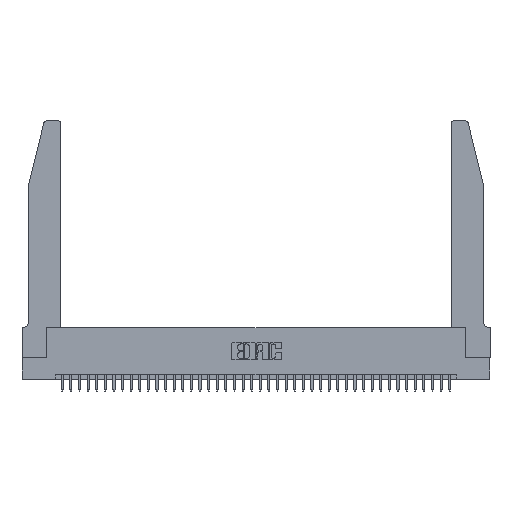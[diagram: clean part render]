
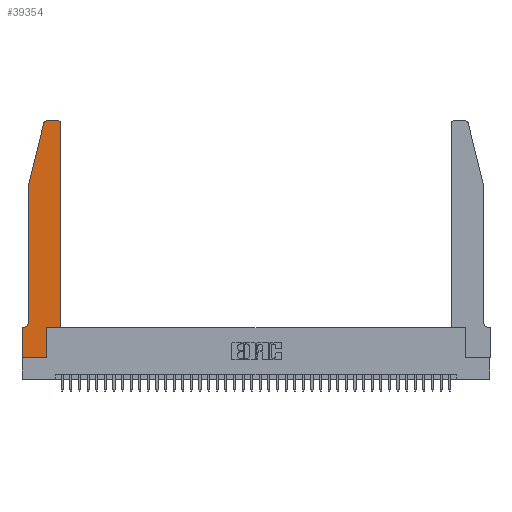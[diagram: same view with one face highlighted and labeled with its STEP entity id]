
A CAD part, top view. The second image highlights one B-rep face of the part: STEP entity #39354.
In plain terms, the highlighted planar face has unit normal (0, 0, 1).
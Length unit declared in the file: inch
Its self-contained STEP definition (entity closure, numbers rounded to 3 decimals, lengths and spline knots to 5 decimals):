
#52 = CARTESIAN_POINT ( 'NONE',  ( 0.4505, 2.72, 0.37 ) ) ;
#160 = VECTOR ( 'NONE', #38831, 39.37008 ) ;
#640 = CARTESIAN_POINT ( 'NONE',  ( 0., 0., 0.37 ) ) ;
#1344 = EDGE_CURVE ( 'NONE', #25017, #6394, #32890, .T. ) ;
#1852 = EDGE_CURVE ( 'NONE', #9838, #25017, #10891, .T. ) ;
#1958 = VERTEX_POINT ( 'NONE', #5887 ) ;
#1980 = CARTESIAN_POINT ( 'NONE',  ( 0.4505, 0.35, 0.37 ) ) ;
#2454 = EDGE_CURVE ( 'NONE', #7672, #1958, #29952, .T. ) ;
#2679 = VECTOR ( 'NONE', #15431, 39.37008 ) ;
#3601 = CIRCLE ( 'NONE', #31686, 0.07 ) ;
#4180 = CARTESIAN_POINT ( 'NONE',  ( 0.25487, 2.72718, 0.37 ) ) ;
#4517 = LINE ( 'NONE', #11717, #35699 ) ;
#4540 = VERTEX_POINT ( 'NONE', #34267 ) ;
#4733 = CARTESIAN_POINT ( 'NONE',  ( 0., 0., 0.37 ) ) ;
#5561 = ORIENTED_EDGE ( 'NONE', *, *, #21082, .T. ) ;
#5887 = CARTESIAN_POINT ( 'NONE',  ( 0.2865, 0.35, 0.37 ) ) ;
#6394 = VERTEX_POINT ( 'NONE', #34773 ) ;
#6833 = ORIENTED_EDGE ( 'NONE', *, *, #37310, .T. ) ;
#6899 = ORIENTED_EDGE ( 'NONE', *, *, #2454, .T. ) ;
#6963 = CARTESIAN_POINT ( 'NONE',  ( 0.0755, 0.35, 0.37 ) ) ;
#7026 = DIRECTION ( 'NONE',  ( 0., 0., 1. ) ) ;
#7358 = DIRECTION ( 'NONE',  ( 0., 1., 0. ) ) ;
#7595 = VECTOR ( 'NONE', #39859, 39.37008 ) ;
#7672 = VERTEX_POINT ( 'NONE', #20774 ) ;
#7779 = VERTEX_POINT ( 'NONE', #36975 ) ;
#7908 = EDGE_LOOP ( 'NONE', ( #13437, #30559, #15495, #39359, #20787, #9068, #5561, #25976, #6899, #21098, #26045, #6833 ) ) ;
#8814 = VECTOR ( 'NONE', #17128, 39.37008 ) ;
#9041 = DIRECTION ( 'NONE',  ( 1., 0., 0. ) ) ;
#9068 = ORIENTED_EDGE ( 'NONE', *, *, #19324, .T. ) ;
#9171 = CARTESIAN_POINT ( 'NONE',  ( 0.4205, 2.72, 0.37 ) ) ;
#9838 = VERTEX_POINT ( 'NONE', #30377 ) ;
#10891 = CIRCLE ( 'NONE', #25066, 0.03 ) ;
#11016 = AXIS2_PLACEMENT_3D ( 'NONE', #9171, #28280, #24979 ) ;
#11222 = DIRECTION ( 'NONE',  ( 0., 0., -1. ) ) ;
#11717 = CARTESIAN_POINT ( 'NONE',  ( 0.4505, 0.35, 0.37 ) ) ;
#11773 = VERTEX_POINT ( 'NONE', #640 ) ;
#12362 = CIRCLE ( 'NONE', #11016, 0.03 ) ;
#13437 = ORIENTED_EDGE ( 'NONE', *, *, #26043, .T. ) ;
#13748 = VECTOR ( 'NONE', #23115, 39.37008 ) ;
#13892 = VECTOR ( 'NONE', #7358, 39.37008 ) ;
#14963 = EDGE_CURVE ( 'NONE', #4540, #35658, #40292, .T. ) ;
#15431 = DIRECTION ( 'NONE',  ( -0.239, -0.971, 0. ) ) ;
#15495 = ORIENTED_EDGE ( 'NONE', *, *, #1344, .T. ) ;
#15550 = VECTOR ( 'NONE', #21327, 39.37008 ) ;
#15794 = CARTESIAN_POINT ( 'NONE',  ( 0.0755, 2., 0.37 ) ) ;
#16838 = CARTESIAN_POINT ( 'NONE',  ( 0., 0.35, 0.37 ) ) ;
#17128 = DIRECTION ( 'NONE',  ( 1., 0., 0. ) ) ;
#18031 = LINE ( 'NONE', #6963, #38524 ) ;
#18348 = VERTEX_POINT ( 'NONE', #18523 ) ;
#18523 = CARTESIAN_POINT ( 'NONE',  ( 0.0055, 0.35, 0.37 ) ) ;
#19031 = VERTEX_POINT ( 'NONE', #32284 ) ;
#19324 = EDGE_CURVE ( 'NONE', #18348, #19031, #18031, .T. ) ;
#19551 = DIRECTION ( 'NONE',  ( 1., 0., 0. ) ) ;
#20001 = CARTESIAN_POINT ( 'NONE',  ( 0.2605, 2.75, 0.37 ) ) ;
#20774 = CARTESIAN_POINT ( 'NONE',  ( 0.2865, 0., 0.37 ) ) ;
#20787 = ORIENTED_EDGE ( 'NONE', *, *, #38173, .T. ) ;
#21021 = CARTESIAN_POINT ( 'NONE',  ( 0.0055, 0.42, 0.37 ) ) ;
#21082 = EDGE_CURVE ( 'NONE', #19031, #11773, #25913, .T. ) ;
#21098 = ORIENTED_EDGE ( 'NONE', *, *, #39048, .T. ) ;
#21327 = DIRECTION ( 'NONE',  ( 0., -1., 0. ) ) ;
#22355 = CARTESIAN_POINT ( 'NONE',  ( 0.2865, 0.35, 0.37 ) ) ;
#23115 = DIRECTION ( 'NONE',  ( 0., -1., 0. ) ) ;
#23856 = LINE ( 'NONE', #33466, #15550 ) ;
#24187 = AXIS2_PLACEMENT_3D ( 'NONE', #16838, #7026, #19551 ) ;
#24648 = DIRECTION ( 'NONE',  ( 1., 0., 0. ) ) ;
#24979 = DIRECTION ( 'NONE',  ( 1., 0., 0. ) ) ;
#25017 = VERTEX_POINT ( 'NONE', #4180 ) ;
#25066 = AXIS2_PLACEMENT_3D ( 'NONE', #25802, #35178, #9041 ) ;
#25802 = CARTESIAN_POINT ( 'NONE',  ( 0.284, 2.72, 0.37 ) ) ;
#25913 = LINE ( 'NONE', #4733, #13748 ) ;
#25976 = ORIENTED_EDGE ( 'NONE', *, *, #34323, .T. ) ;
#26003 = CARTESIAN_POINT ( 'NONE',  ( 0., 0., 0.37 ) ) ;
#26043 = EDGE_CURVE ( 'NONE', #30012, #9838, #34295, .T. ) ;
#26045 = ORIENTED_EDGE ( 'NONE', *, *, #14963, .T. ) ;
#27066 = DIRECTION ( 'NONE',  ( -1., 0., 0. ) ) ;
#28280 = DIRECTION ( 'NONE',  ( 0., 0., 1. ) ) ;
#29811 = CARTESIAN_POINT ( 'NONE',  ( 0.4205, 2.75, 0.37 ) ) ;
#29952 = LINE ( 'NONE', #22355, #13892 ) ;
#30012 = VERTEX_POINT ( 'NONE', #29811 ) ;
#30047 = EDGE_CURVE ( 'NONE', #6394, #7779, #23856, .T. ) ;
#30377 = CARTESIAN_POINT ( 'NONE',  ( 0.284, 2.75, 0.37 ) ) ;
#30559 = ORIENTED_EDGE ( 'NONE', *, *, #1852, .T. ) ;
#31686 = AXIS2_PLACEMENT_3D ( 'NONE', #21021, #11222, #27066 ) ;
#32284 = CARTESIAN_POINT ( 'NONE',  ( 0., 0.35, 0.37 ) ) ;
#32890 = LINE ( 'NONE', #15794, #2679 ) ;
#33466 = CARTESIAN_POINT ( 'NONE',  ( 0.0755, 2., 0.37 ) ) ;
#34267 = CARTESIAN_POINT ( 'NONE',  ( 0.4505, 0.35, 0.37 ) ) ;
#34295 = LINE ( 'NONE', #20001, #160 ) ;
#34323 = EDGE_CURVE ( 'NONE', #11773, #7672, #36126, .T. ) ;
#34773 = CARTESIAN_POINT ( 'NONE',  ( 0.0755, 2., 0.37 ) ) ;
#34889 = DIRECTION ( 'NONE',  ( -1., 0., 0. ) ) ;
#35178 = DIRECTION ( 'NONE',  ( 0., 0., 1. ) ) ;
#35508 = PLANE ( 'NONE',  #24187 ) ;
#35658 = VERTEX_POINT ( 'NONE', #52 ) ;
#35699 = VECTOR ( 'NONE', #24648, 39.37008 ) ;
#36126 = LINE ( 'NONE', #26003, #8814 ) ;
#36975 = CARTESIAN_POINT ( 'NONE',  ( 0.0755, 0.42, 0.37 ) ) ;
#37310 = EDGE_CURVE ( 'NONE', #35658, #30012, #12362, .T. ) ;
#38173 = EDGE_CURVE ( 'NONE', #7779, #18348, #3601, .T. ) ;
#38524 = VECTOR ( 'NONE', #34889, 39.37008 ) ;
#38594 = FACE_OUTER_BOUND ( 'NONE', #7908, .T. ) ;
#38831 = DIRECTION ( 'NONE',  ( -1., 0., 0. ) ) ;
#39048 = EDGE_CURVE ( 'NONE', #1958, #4540, #4517, .T. ) ;
#39354 = ADVANCED_FACE ( 'NONE', ( #38594 ), #35508, .T. ) ;
#39359 = ORIENTED_EDGE ( 'NONE', *, *, #30047, .T. ) ;
#39859 = DIRECTION ( 'NONE',  ( 0., 1., 0. ) ) ;
#40292 = LINE ( 'NONE', #1980, #7595 ) ;
